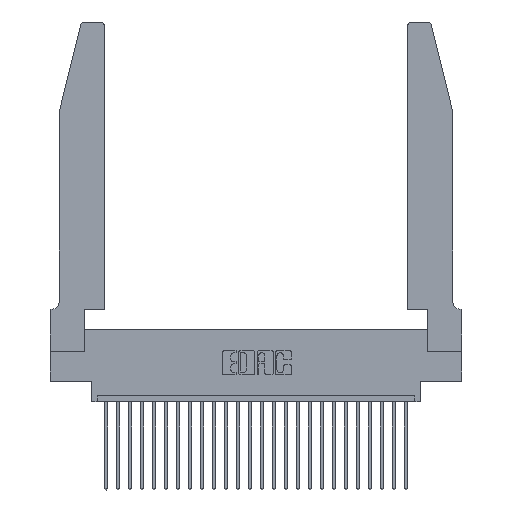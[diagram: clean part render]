
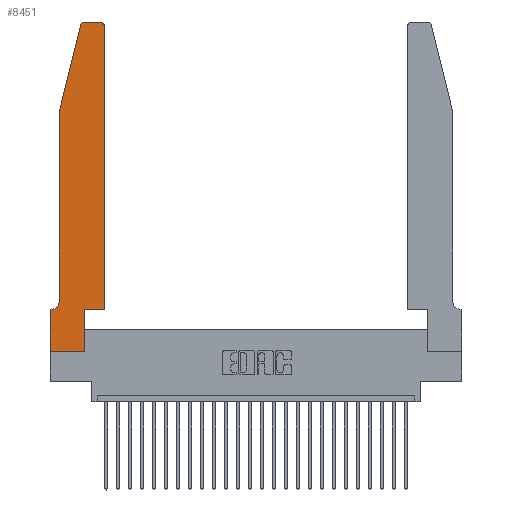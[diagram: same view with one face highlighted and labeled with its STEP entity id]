
A CAD part, top view. The second image highlights one B-rep face of the part: STEP entity #8451.
In plain terms, the highlighted planar face has unit normal (0, 0, 1).
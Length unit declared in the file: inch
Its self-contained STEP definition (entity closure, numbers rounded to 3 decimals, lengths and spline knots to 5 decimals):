
#845 = LINE ( 'NONE', #13350, #16845 ) ;
#1311 = LINE ( 'NONE', #14983, #18934 ) ;
#1832 = DIRECTION ( 'NONE',  ( 0., 0., 1. ) ) ;
#1885 = AXIS2_PLACEMENT_3D ( 'NONE', #21715, #23878, #11798 ) ;
#2204 = CARTESIAN_POINT ( 'NONE',  ( 0.2865, 0., 0.37 ) ) ;
#2589 = EDGE_CURVE ( 'NONE', #12545, #23289, #5529, .T. ) ;
#2781 = DIRECTION ( 'NONE',  ( 1., 0., 0. ) ) ;
#2988 = DIRECTION ( 'NONE',  ( 0., 0., -1. ) ) ;
#3402 = ORIENTED_EDGE ( 'NONE', *, *, #18120, .T. ) ;
#3616 = ORIENTED_EDGE ( 'NONE', *, *, #26482, .T. ) ;
#3834 = CARTESIAN_POINT ( 'NONE',  ( 0.4505, 2.72, 0.37 ) ) ;
#3929 = DIRECTION ( 'NONE',  ( 0., -1., 0. ) ) ;
#4079 = EDGE_CURVE ( 'NONE', #22713, #18776, #1311, .T. ) ;
#4269 = EDGE_CURVE ( 'NONE', #24265, #23181, #24393, .T. ) ;
#4895 = CARTESIAN_POINT ( 'NONE',  ( 0.4505, 0.35, 0.37 ) ) ;
#5006 = LINE ( 'NONE', #22234, #26237 ) ;
#5064 = DIRECTION ( 'NONE',  ( 0., 0., 1. ) ) ;
#5163 = DIRECTION ( 'NONE',  ( 0., 1., 0. ) ) ;
#5216 = EDGE_CURVE ( 'NONE', #11213, #22713, #9599, .T. ) ;
#5466 = CARTESIAN_POINT ( 'NONE',  ( 0.0055, 0.35, 0.37 ) ) ;
#5529 = LINE ( 'NONE', #14034, #20968 ) ;
#5938 = CARTESIAN_POINT ( 'NONE',  ( 0., 0., 0.37 ) ) ;
#6328 = VECTOR ( 'NONE', #20052, 39.37008 ) ;
#6436 = EDGE_CURVE ( 'NONE', #20112, #18362, #21749, .T. ) ;
#6583 = ORIENTED_EDGE ( 'NONE', *, *, #4269, .T. ) ;
#7439 = CARTESIAN_POINT ( 'NONE',  ( 0.2865, 0.35, 0.37 ) ) ;
#7449 = ORIENTED_EDGE ( 'NONE', *, *, #2589, .T. ) ;
#7870 = CARTESIAN_POINT ( 'NONE',  ( 0.0755, 0.35, 0.37 ) ) ;
#8247 = VECTOR ( 'NONE', #18006, 39.37008 ) ;
#8451 = ADVANCED_FACE ( 'NONE', ( #8774 ), #19151, .T. ) ;
#8543 = LINE ( 'NONE', #26109, #12702 ) ;
#8774 = FACE_OUTER_BOUND ( 'NONE', #12478, .T. ) ;
#8918 = DIRECTION ( 'NONE',  ( 0., -1., 0. ) ) ;
#9009 = CARTESIAN_POINT ( 'NONE',  ( 0.0755, 0.42, 0.37 ) ) ;
#9284 = ORIENTED_EDGE ( 'NONE', *, *, #5216, .T. ) ;
#9599 = LINE ( 'NONE', #7870, #18879 ) ;
#10050 = CARTESIAN_POINT ( 'NONE',  ( 0.4505, 0.35, 0.37 ) ) ;
#10195 = EDGE_CURVE ( 'NONE', #18362, #10341, #845, .T. ) ;
#10341 = VERTEX_POINT ( 'NONE', #10050 ) ;
#10461 = ORIENTED_EDGE ( 'NONE', *, *, #22428, .T. ) ;
#10535 = CARTESIAN_POINT ( 'NONE',  ( 0.2865, 0.35, 0.37 ) ) ;
#11213 = VERTEX_POINT ( 'NONE', #5466 ) ;
#11320 = ORIENTED_EDGE ( 'NONE', *, *, #16438, .T. ) ;
#11377 = CARTESIAN_POINT ( 'NONE',  ( 0.0055, 0.42, 0.37 ) ) ;
#11798 = DIRECTION ( 'NONE',  ( 1., 0., 0. ) ) ;
#11958 = LINE ( 'NONE', #4895, #21309 ) ;
#12056 = ORIENTED_EDGE ( 'NONE', *, *, #6436, .T. ) ;
#12411 = CIRCLE ( 'NONE', #20378, 0.07 ) ;
#12478 = EDGE_LOOP ( 'NONE', ( #11320, #6583, #3402, #7449, #23229, #9284, #16270, #3616, #12056, #25315, #13837, #10461 ) ) ;
#12545 = VERTEX_POINT ( 'NONE', #21116 ) ;
#12702 = VECTOR ( 'NONE', #19987, 39.37008 ) ;
#13347 = AXIS2_PLACEMENT_3D ( 'NONE', #13727, #1832, #13824 ) ;
#13350 = CARTESIAN_POINT ( 'NONE',  ( 0.4505, 0.35, 0.37 ) ) ;
#13727 = CARTESIAN_POINT ( 'NONE',  ( 0.284, 2.72, 0.37 ) ) ;
#13824 = DIRECTION ( 'NONE',  ( 1., 0., 0. ) ) ;
#13837 = ORIENTED_EDGE ( 'NONE', *, *, #22737, .T. ) ;
#14034 = CARTESIAN_POINT ( 'NONE',  ( 0.0755, 2., 0.37 ) ) ;
#14902 = VERTEX_POINT ( 'NONE', #17045 ) ;
#14934 = AXIS2_PLACEMENT_3D ( 'NONE', #25462, #5064, #19434 ) ;
#14983 = CARTESIAN_POINT ( 'NONE',  ( 0., 0., 0.37 ) ) ;
#15287 = CARTESIAN_POINT ( 'NONE',  ( 0., 0.35, 0.37 ) ) ;
#15418 = DIRECTION ( 'NONE',  ( -1., 0., 0. ) ) ;
#15838 = CIRCLE ( 'NONE', #1885, 0.03 ) ;
#16270 = ORIENTED_EDGE ( 'NONE', *, *, #4079, .T. ) ;
#16438 = EDGE_CURVE ( 'NONE', #14902, #24265, #17592, .T. ) ;
#16845 = VECTOR ( 'NONE', #2781, 39.37008 ) ;
#17045 = CARTESIAN_POINT ( 'NONE',  ( 0.4205, 2.75, 0.37 ) ) ;
#17592 = LINE ( 'NONE', #20158, #6328 ) ;
#18006 = DIRECTION ( 'NONE',  ( 0., 1., 0. ) ) ;
#18120 = EDGE_CURVE ( 'NONE', #23181, #12545, #5006, .T. ) ;
#18128 = VERTEX_POINT ( 'NONE', #3834 ) ;
#18362 = VERTEX_POINT ( 'NONE', #10535 ) ;
#18776 = VERTEX_POINT ( 'NONE', #5938 ) ;
#18879 = VECTOR ( 'NONE', #21956, 39.37008 ) ;
#18934 = VECTOR ( 'NONE', #8918, 39.37008 ) ;
#19151 = PLANE ( 'NONE',  #14934 ) ;
#19224 = CARTESIAN_POINT ( 'NONE',  ( 0.25487, 2.72718, 0.37 ) ) ;
#19434 = DIRECTION ( 'NONE',  ( 1., 0., 0. ) ) ;
#19987 = DIRECTION ( 'NONE',  ( 1., 0., 0. ) ) ;
#20052 = DIRECTION ( 'NONE',  ( -1., 0., 0. ) ) ;
#20112 = VERTEX_POINT ( 'NONE', #2204 ) ;
#20158 = CARTESIAN_POINT ( 'NONE',  ( 0.2605, 2.75, 0.37 ) ) ;
#20358 = DIRECTION ( 'NONE',  ( -0.239, -0.971, 0. ) ) ;
#20378 = AXIS2_PLACEMENT_3D ( 'NONE', #11377, #2988, #15418 ) ;
#20806 = CARTESIAN_POINT ( 'NONE',  ( 0.284, 2.75, 0.37 ) ) ;
#20968 = VECTOR ( 'NONE', #3929, 39.37008 ) ;
#21116 = CARTESIAN_POINT ( 'NONE',  ( 0.0755, 2., 0.37 ) ) ;
#21309 = VECTOR ( 'NONE', #5163, 39.37008 ) ;
#21715 = CARTESIAN_POINT ( 'NONE',  ( 0.4205, 2.72, 0.37 ) ) ;
#21749 = LINE ( 'NONE', #7439, #8247 ) ;
#21956 = DIRECTION ( 'NONE',  ( -1., 0., 0. ) ) ;
#22234 = CARTESIAN_POINT ( 'NONE',  ( 0.0755, 2., 0.37 ) ) ;
#22428 = EDGE_CURVE ( 'NONE', #18128, #14902, #15838, .T. ) ;
#22713 = VERTEX_POINT ( 'NONE', #15287 ) ;
#22737 = EDGE_CURVE ( 'NONE', #10341, #18128, #11958, .T. ) ;
#23181 = VERTEX_POINT ( 'NONE', #19224 ) ;
#23229 = ORIENTED_EDGE ( 'NONE', *, *, #25636, .T. ) ;
#23289 = VERTEX_POINT ( 'NONE', #9009 ) ;
#23878 = DIRECTION ( 'NONE',  ( 0., 0., 1. ) ) ;
#24265 = VERTEX_POINT ( 'NONE', #20806 ) ;
#24393 = CIRCLE ( 'NONE', #13347, 0.03 ) ;
#25315 = ORIENTED_EDGE ( 'NONE', *, *, #10195, .T. ) ;
#25462 = CARTESIAN_POINT ( 'NONE',  ( 0., 0.35, 0.37 ) ) ;
#25636 = EDGE_CURVE ( 'NONE', #23289, #11213, #12411, .T. ) ;
#26109 = CARTESIAN_POINT ( 'NONE',  ( 0., 0., 0.37 ) ) ;
#26237 = VECTOR ( 'NONE', #20358, 39.37008 ) ;
#26482 = EDGE_CURVE ( 'NONE', #18776, #20112, #8543, .T. ) ;
